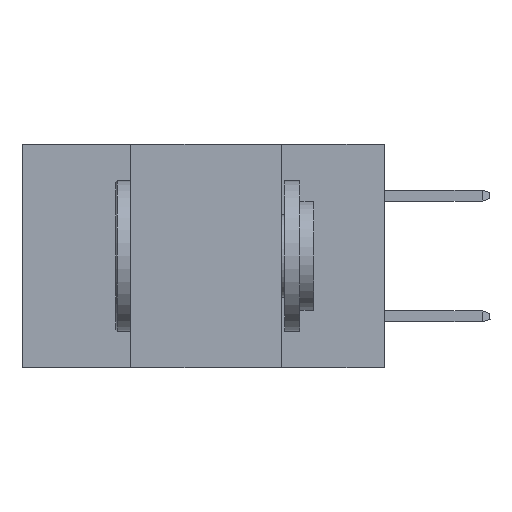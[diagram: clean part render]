
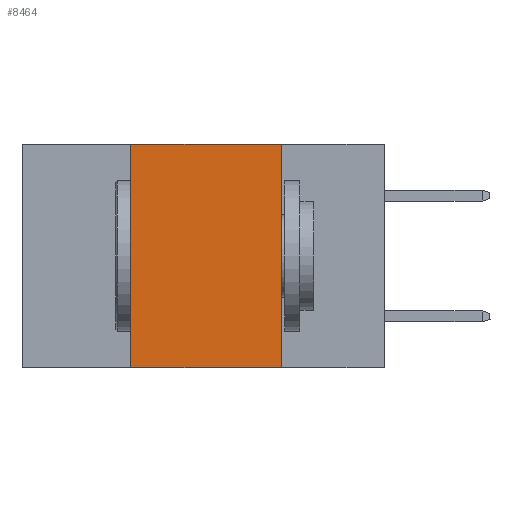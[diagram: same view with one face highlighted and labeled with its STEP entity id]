
A CAD part, left-side view. The second image highlights one B-rep face of the part: STEP entity #8464.
In plain terms, the highlighted planar face has unit normal (-1, 0, 0).
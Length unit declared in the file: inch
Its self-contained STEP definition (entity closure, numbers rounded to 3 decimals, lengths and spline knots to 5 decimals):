
#529 = VERTEX_POINT ( 'NONE', #12476 ) ;
#1142 = DIRECTION ( 'NONE',  ( 0., 0., -1. ) ) ;
#1551 = CARTESIAN_POINT ( 'NONE',  ( 0., 0.6, 0. ) ) ;
#1873 = VECTOR ( 'NONE', #5731, 39.37008 ) ;
#2910 = AXIS2_PLACEMENT_3D ( 'NONE', #7344, #13445, #1142 ) ;
#3241 = CARTESIAN_POINT ( 'NONE',  ( 0., 0.17, -0.37 ) ) ;
#3415 = DIRECTION ( 'NONE',  ( 0., -1., 0. ) ) ;
#3469 = CARTESIAN_POINT ( 'NONE',  ( 0., 0.17, -0.37 ) ) ;
#4165 = EDGE_CURVE ( 'NONE', #15850, #8644, #16166, .T. ) ;
#4751 = VECTOR ( 'NONE', #5279, 39.37008 ) ;
#4968 = VERTEX_POINT ( 'NONE', #3469 ) ;
#5279 = DIRECTION ( 'NONE',  ( 0., 0., -1. ) ) ;
#5482 = ORIENTED_EDGE ( 'NONE', *, *, #4165, .F. ) ;
#5731 = DIRECTION ( 'NONE',  ( 0., -1., 0. ) ) ;
#6042 = LINE ( 'NONE', #3241, #4751 ) ;
#6131 = ORIENTED_EDGE ( 'NONE', *, *, #16540, .T. ) ;
#7344 = CARTESIAN_POINT ( 'NONE',  ( 0., 0.6, 0. ) ) ;
#7759 = DIRECTION ( 'NONE',  ( 0., 0., 1. ) ) ;
#7990 = CARTESIAN_POINT ( 'NONE',  ( 0., 0.42, -0.37 ) ) ;
#8464 = ADVANCED_FACE ( 'NONE', ( #17987 ), #11442, .F. ) ;
#8644 = VERTEX_POINT ( 'NONE', #16017 ) ;
#9647 = ORIENTED_EDGE ( 'NONE', *, *, #18300, .F. ) ;
#9967 = LINE ( 'NONE', #19563, #25386 ) ;
#11042 = EDGE_LOOP ( 'NONE', ( #9647, #21018, #5482, #6131 ) ) ;
#11442 = PLANE ( 'NONE',  #2910 ) ;
#12476 = CARTESIAN_POINT ( 'NONE',  ( 0., 0.17, 0. ) ) ;
#13445 = DIRECTION ( 'NONE',  ( 1., 0., 0. ) ) ;
#15850 = VERTEX_POINT ( 'NONE', #21649 ) ;
#16017 = CARTESIAN_POINT ( 'NONE',  ( 0., 0.42, 0. ) ) ;
#16166 = LINE ( 'NONE', #7990, #20257 ) ;
#16540 = EDGE_CURVE ( 'NONE', #15850, #4968, #9967, .T. ) ;
#16629 = EDGE_CURVE ( 'NONE', #8644, #529, #18157, .T. ) ;
#17987 = FACE_OUTER_BOUND ( 'NONE', #11042, .T. ) ;
#18157 = LINE ( 'NONE', #1551, #1873 ) ;
#18300 = EDGE_CURVE ( 'NONE', #529, #4968, #6042, .T. ) ;
#19563 = CARTESIAN_POINT ( 'NONE',  ( 0., 0.6, -0.37 ) ) ;
#20257 = VECTOR ( 'NONE', #7759, 39.37008 ) ;
#21018 = ORIENTED_EDGE ( 'NONE', *, *, #16629, .F. ) ;
#21649 = CARTESIAN_POINT ( 'NONE',  ( 0., 0.42, -0.37 ) ) ;
#25386 = VECTOR ( 'NONE', #3415, 39.37008 ) ;
